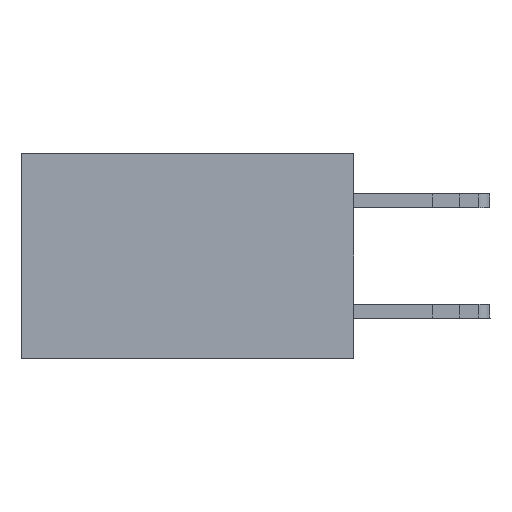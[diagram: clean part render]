
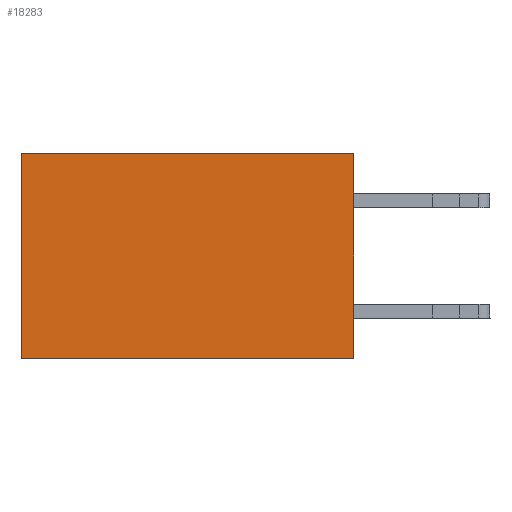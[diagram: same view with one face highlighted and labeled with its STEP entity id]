
A CAD part, left-side view. The second image highlights one B-rep face of the part: STEP entity #18283.
In plain terms, the highlighted planar face has unit normal (-1, 0, 0).
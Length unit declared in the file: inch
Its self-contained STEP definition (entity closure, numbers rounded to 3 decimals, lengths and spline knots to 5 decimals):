
#154 = VECTOR ( 'NONE', #764, 39.37008 ) ;
#185 = EDGE_LOOP ( 'NONE', ( #26143, #25268, #25256, #30975 ) ) ;
#764 = DIRECTION ( 'NONE',  ( 0., 1., 0. ) ) ;
#2602 = CARTESIAN_POINT ( 'NONE',  ( 0.2875, 0., -0.37 ) ) ;
#2966 = VERTEX_POINT ( 'NONE', #16608 ) ;
#3663 = CARTESIAN_POINT ( 'NONE',  ( 0.2875, 0.6, -0.37 ) ) ;
#5543 = DIRECTION ( 'NONE',  ( 1., 0., 0. ) ) ;
#6566 = VERTEX_POINT ( 'NONE', #26416 ) ;
#7900 = DIRECTION ( 'NONE',  ( 0., 0., -1. ) ) ;
#10359 = PLANE ( 'NONE',  #17906 ) ;
#11341 = VECTOR ( 'NONE', #16175, 39.37008 ) ;
#11391 = EDGE_CURVE ( 'NONE', #16165, #15462, #25410, .T. ) ;
#13066 = CARTESIAN_POINT ( 'NONE',  ( 0.2875, 0., 0. ) ) ;
#14055 = EDGE_CURVE ( 'NONE', #6566, #15462, #32918, .T. ) ;
#14435 = VECTOR ( 'NONE', #20977, 39.37008 ) ;
#15462 = VERTEX_POINT ( 'NONE', #3663 ) ;
#16165 = VERTEX_POINT ( 'NONE', #19542 ) ;
#16175 = DIRECTION ( 'NONE',  ( 0., 1., 0. ) ) ;
#16608 = CARTESIAN_POINT ( 'NONE',  ( 0.2875, 0., 0. ) ) ;
#17297 = CARTESIAN_POINT ( 'NONE',  ( 0.2875, 0.6, 0. ) ) ;
#17906 = AXIS2_PLACEMENT_3D ( 'NONE', #13066, #5543, #7900 ) ;
#18283 = ADVANCED_FACE ( 'NONE', ( #26237 ), #10359, .F. ) ;
#19542 = CARTESIAN_POINT ( 'NONE',  ( 0.2875, 0., -0.37 ) ) ;
#19782 = DIRECTION ( 'NONE',  ( 0., 0., -1. ) ) ;
#20977 = DIRECTION ( 'NONE',  ( 0., 0., -1. ) ) ;
#21196 = CARTESIAN_POINT ( 'NONE',  ( 0.2875, 0., 0. ) ) ;
#25256 = ORIENTED_EDGE ( 'NONE', *, *, #25933, .F. ) ;
#25268 = ORIENTED_EDGE ( 'NONE', *, *, #11391, .F. ) ;
#25410 = LINE ( 'NONE', #2602, #11341 ) ;
#25670 = LINE ( 'NONE', #21196, #14435 ) ;
#25933 = EDGE_CURVE ( 'NONE', #2966, #16165, #25670, .T. ) ;
#26143 = ORIENTED_EDGE ( 'NONE', *, *, #14055, .T. ) ;
#26237 = FACE_OUTER_BOUND ( 'NONE', #185, .T. ) ;
#26277 = CARTESIAN_POINT ( 'NONE',  ( 0.2875, 0., 0. ) ) ;
#26416 = CARTESIAN_POINT ( 'NONE',  ( 0.2875, 0.6, 0. ) ) ;
#28401 = EDGE_CURVE ( 'NONE', #2966, #6566, #30268, .T. ) ;
#29703 = VECTOR ( 'NONE', #19782, 39.37008 ) ;
#30268 = LINE ( 'NONE', #26277, #154 ) ;
#30975 = ORIENTED_EDGE ( 'NONE', *, *, #28401, .T. ) ;
#32918 = LINE ( 'NONE', #17297, #29703 ) ;
